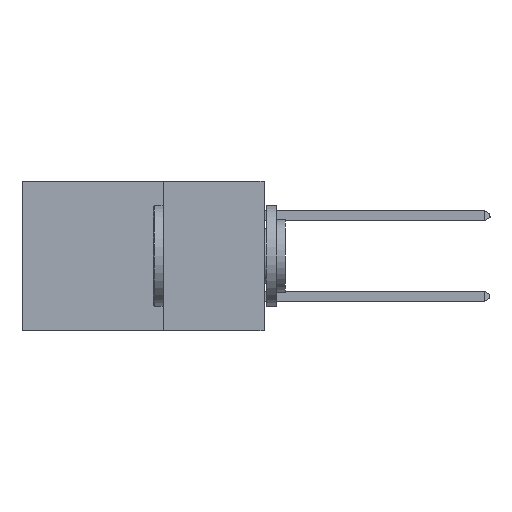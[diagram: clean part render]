
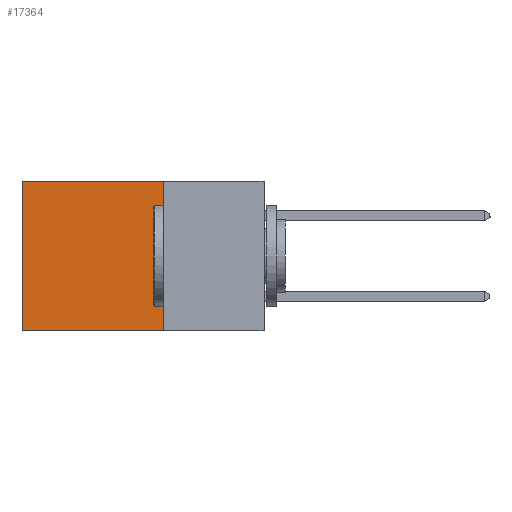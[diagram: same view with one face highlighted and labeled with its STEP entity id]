
A CAD part, left-side view. The second image highlights one B-rep face of the part: STEP entity #17364.
In plain terms, the highlighted planar face has unit normal (-1, 0, 0).
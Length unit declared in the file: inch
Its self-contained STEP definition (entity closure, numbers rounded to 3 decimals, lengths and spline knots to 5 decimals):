
#619 = VECTOR ( 'NONE', #5499, 39.37008 ) ;
#1428 = EDGE_CURVE ( 'NONE', #15584, #10605, #12589, .T. ) ;
#1614 = DIRECTION ( 'NONE',  ( 1., 0., 0. ) ) ;
#1824 = AXIS2_PLACEMENT_3D ( 'NONE', #10272, #1614, #13828 ) ;
#3325 = VECTOR ( 'NONE', #14800, 39.37008 ) ;
#3764 = CARTESIAN_POINT ( 'NONE',  ( 0.298, 0.25, 0. ) ) ;
#3860 = VECTOR ( 'NONE', #20522, 39.37008 ) ;
#3887 = LINE ( 'NONE', #18155, #3325 ) ;
#4479 = DIRECTION ( 'NONE',  ( 0., 0., -1. ) ) ;
#4988 = CARTESIAN_POINT ( 'NONE',  ( 0.298, 0.25, 0. ) ) ;
#5257 = LINE ( 'NONE', #3764, #619 ) ;
#5499 = DIRECTION ( 'NONE',  ( 0., 1., 0. ) ) ;
#5687 = CARTESIAN_POINT ( 'NONE',  ( 0.298, 0.6, -0.37 ) ) ;
#6332 = EDGE_LOOP ( 'NONE', ( #9613, #20042, #11321, #9182 ) ) ;
#8063 = VERTEX_POINT ( 'NONE', #4988 ) ;
#8807 = VECTOR ( 'NONE', #4479, 39.37008 ) ;
#8982 = CARTESIAN_POINT ( 'NONE',  ( 0.298, 0.25, -0.37 ) ) ;
#9182 = ORIENTED_EDGE ( 'NONE', *, *, #15580, .T. ) ;
#9613 = ORIENTED_EDGE ( 'NONE', *, *, #10689, .T. ) ;
#9841 = FACE_OUTER_BOUND ( 'NONE', #6332, .T. ) ;
#10272 = CARTESIAN_POINT ( 'NONE',  ( 0.298, 0.25, 0. ) ) ;
#10605 = VERTEX_POINT ( 'NONE', #5687 ) ;
#10689 = EDGE_CURVE ( 'NONE', #20262, #10605, #3887, .T. ) ;
#11321 = ORIENTED_EDGE ( 'NONE', *, *, #16531, .F. ) ;
#12589 = LINE ( 'NONE', #22228, #3860 ) ;
#12862 = LINE ( 'NONE', #14890, #8807 ) ;
#13828 = DIRECTION ( 'NONE',  ( 0., 0., -1. ) ) ;
#14800 = DIRECTION ( 'NONE',  ( 0., 0., -1. ) ) ;
#14890 = CARTESIAN_POINT ( 'NONE',  ( 0.298, 0.25, 0. ) ) ;
#15479 = PLANE ( 'NONE',  #1824 ) ;
#15580 = EDGE_CURVE ( 'NONE', #8063, #20262, #5257, .T. ) ;
#15584 = VERTEX_POINT ( 'NONE', #8982 ) ;
#16531 = EDGE_CURVE ( 'NONE', #8063, #15584, #12862, .T. ) ;
#17364 = ADVANCED_FACE ( 'NONE', ( #9841 ), #15479, .F. ) ;
#17511 = CARTESIAN_POINT ( 'NONE',  ( 0.298, 0.6, 0. ) ) ;
#18155 = CARTESIAN_POINT ( 'NONE',  ( 0.298, 0.6, 0. ) ) ;
#20042 = ORIENTED_EDGE ( 'NONE', *, *, #1428, .F. ) ;
#20262 = VERTEX_POINT ( 'NONE', #17511 ) ;
#20522 = DIRECTION ( 'NONE',  ( 0., 1., 0. ) ) ;
#22228 = CARTESIAN_POINT ( 'NONE',  ( 0.298, 0.25, -0.37 ) ) ;
